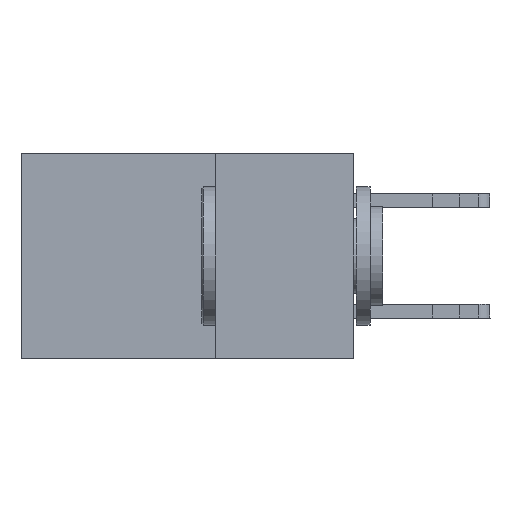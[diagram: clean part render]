
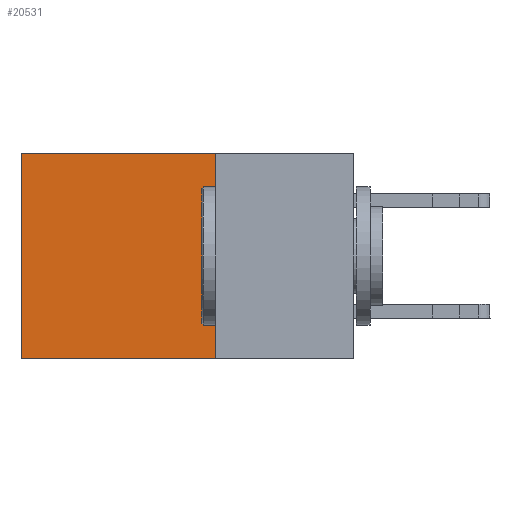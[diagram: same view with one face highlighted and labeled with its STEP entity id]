
A CAD part, left-side view. The second image highlights one B-rep face of the part: STEP entity #20531.
In plain terms, the highlighted planar face has unit normal (-1, 0, 0).
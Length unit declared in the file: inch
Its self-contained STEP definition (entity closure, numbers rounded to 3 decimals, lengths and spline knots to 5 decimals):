
#308 = VECTOR ( 'NONE', #1323, 39.37008 ) ;
#849 = CARTESIAN_POINT ( 'NONE',  ( 0.2875, 0.6, 0. ) ) ;
#1323 = DIRECTION ( 'NONE',  ( 0., 1., 0. ) ) ;
#1916 = CARTESIAN_POINT ( 'NONE',  ( 0.2875, 0.25, 0. ) ) ;
#2021 = PLANE ( 'NONE',  #7470 ) ;
#3321 = EDGE_CURVE ( 'NONE', #20945, #25906, #19035, .T. ) ;
#3329 = VECTOR ( 'NONE', #15529, 39.37008 ) ;
#3571 = CARTESIAN_POINT ( 'NONE',  ( 0.2875, 0.25, 0. ) ) ;
#3634 = EDGE_CURVE ( 'NONE', #23335, #24962, #12521, .T. ) ;
#4080 = CARTESIAN_POINT ( 'NONE',  ( 0.2875, 0.6, -0.37 ) ) ;
#4741 = ORIENTED_EDGE ( 'NONE', *, *, #3321, .F. ) ;
#5184 = CARTESIAN_POINT ( 'NONE',  ( 0.2875, 0.25, -0.37 ) ) ;
#6772 = ORIENTED_EDGE ( 'NONE', *, *, #13620, .F. ) ;
#6822 = FACE_OUTER_BOUND ( 'NONE', #18758, .T. ) ;
#6834 = ORIENTED_EDGE ( 'NONE', *, *, #19560, .T. ) ;
#7242 = CARTESIAN_POINT ( 'NONE',  ( 0.2875, 0.25, -0.37 ) ) ;
#7470 = AXIS2_PLACEMENT_3D ( 'NONE', #16753, #10506, #16670 ) ;
#7848 = DIRECTION ( 'NONE',  ( 0., 1., 0. ) ) ;
#10506 = DIRECTION ( 'NONE',  ( 1., 0., 0. ) ) ;
#12521 = LINE ( 'NONE', #24445, #3329 ) ;
#13620 = EDGE_CURVE ( 'NONE', #25906, #24962, #24125, .T. ) ;
#15529 = DIRECTION ( 'NONE',  ( 0., 0., -1. ) ) ;
#15742 = LINE ( 'NONE', #3571, #19964 ) ;
#16670 = DIRECTION ( 'NONE',  ( 0., 0., -1. ) ) ;
#16753 = CARTESIAN_POINT ( 'NONE',  ( 0.2875, 0.25, 0. ) ) ;
#18758 = EDGE_LOOP ( 'NONE', ( #20881, #6772, #4741, #6834 ) ) ;
#19035 = LINE ( 'NONE', #26827, #25561 ) ;
#19560 = EDGE_CURVE ( 'NONE', #20945, #23335, #15742, .T. ) ;
#19964 = VECTOR ( 'NONE', #7848, 39.37008 ) ;
#20531 = ADVANCED_FACE ( 'NONE', ( #6822 ), #2021, .F. ) ;
#20881 = ORIENTED_EDGE ( 'NONE', *, *, #3634, .T. ) ;
#20945 = VERTEX_POINT ( 'NONE', #1916 ) ;
#23335 = VERTEX_POINT ( 'NONE', #849 ) ;
#24125 = LINE ( 'NONE', #7242, #308 ) ;
#24445 = CARTESIAN_POINT ( 'NONE',  ( 0.2875, 0.6, 0. ) ) ;
#24628 = DIRECTION ( 'NONE',  ( 0., 0., -1. ) ) ;
#24962 = VERTEX_POINT ( 'NONE', #4080 ) ;
#25561 = VECTOR ( 'NONE', #24628, 39.37008 ) ;
#25906 = VERTEX_POINT ( 'NONE', #5184 ) ;
#26827 = CARTESIAN_POINT ( 'NONE',  ( 0.2875, 0.25, 0. ) ) ;
